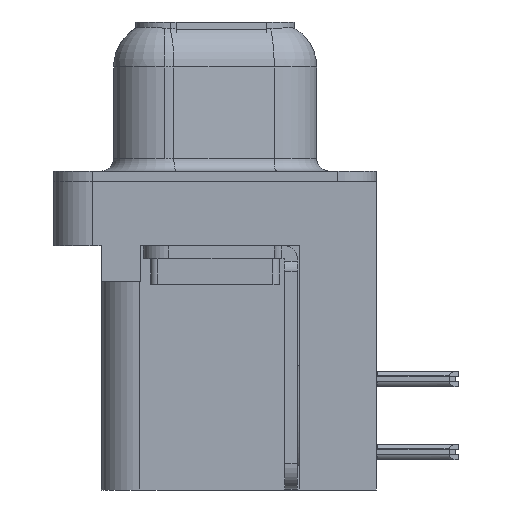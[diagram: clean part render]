
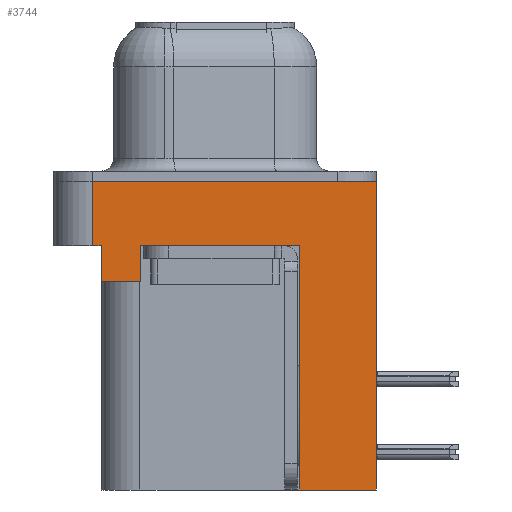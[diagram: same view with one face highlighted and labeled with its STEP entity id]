
A CAD part, left-side view. The second image highlights one B-rep face of the part: STEP entity #3744.
In plain terms, the highlighted planar face has unit normal (-1, 0, 0).
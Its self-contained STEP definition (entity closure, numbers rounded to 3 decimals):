
#469 = VERTEX_POINT ( 'NONE', #25335 ) ;
#672 = VERTEX_POINT ( 'NONE', #24510 ) ;
#760 = CARTESIAN_POINT ( 'NONE',  ( -3., -3.295, -12. ) ) ;
#1376 = CARTESIAN_POINT ( 'NONE',  ( -3., 4.775, -2.5 ) ) ;
#2022 = VECTOR ( 'NONE', #10264, 1000. ) ;
#2305 = LINE ( 'NONE', #1376, #24453 ) ;
#2306 = VECTOR ( 'NONE', #3288, 1000. ) ;
#2767 = LINE ( 'NONE', #17264, #2022 ) ;
#2804 = VERTEX_POINT ( 'NONE', #12885 ) ;
#3288 = DIRECTION ( 'NONE',  ( 0., 0., 1. ) ) ;
#3420 = EDGE_CURVE ( 'NONE', #29786, #469, #21900, .T. ) ;
#3744 = ADVANCED_FACE ( 'NONE', ( #12641 ), #6191, .T. ) ;
#4097 = ORIENTED_EDGE ( 'NONE', *, *, #20333, .F. ) ;
#4648 = CARTESIAN_POINT ( 'NONE',  ( -3., -3.295, -12. ) ) ;
#4680 = VERTEX_POINT ( 'NONE', #21486 ) ;
#5271 = LINE ( 'NONE', #19045, #11168 ) ;
#5850 = EDGE_CURVE ( 'NONE', #29208, #2804, #10130, .T. ) ;
#5971 = ORIENTED_EDGE ( 'NONE', *, *, #20144, .T. ) ;
#6191 = PLANE ( 'NONE',  #15124 ) ;
#6285 = ORIENTED_EDGE ( 'NONE', *, *, #27830, .T. ) ;
#8694 = DIRECTION ( 'NONE',  ( 0., 1., 0. ) ) ;
#8853 = ORIENTED_EDGE ( 'NONE', *, *, #11262, .F. ) ;
#8921 = VECTOR ( 'NONE', #8694, 1000. ) ;
#9347 = DIRECTION ( 'NONE',  ( 0., 0., 1. ) ) ;
#9670 = LINE ( 'NONE', #18084, #8921 ) ;
#10130 = LINE ( 'NONE', #19943, #10865 ) ;
#10264 = DIRECTION ( 'NONE',  ( 0., -1., 0. ) ) ;
#10350 = VERTEX_POINT ( 'NONE', #25648 ) ;
#10865 = VECTOR ( 'NONE', #22659, 1000. ) ;
#11033 = VERTEX_POINT ( 'NONE', #12132 ) ;
#11168 = VECTOR ( 'NONE', #9347, 1000. ) ;
#11219 = EDGE_CURVE ( 'NONE', #10350, #29208, #2305, .T. ) ;
#11262 = EDGE_CURVE ( 'NONE', #4680, #29013, #9670, .T. ) ;
#12012 = CARTESIAN_POINT ( 'NONE',  ( -3., -3.295, -2.5 ) ) ;
#12132 = CARTESIAN_POINT ( 'NONE',  ( -3., 4.425, -2.5 ) ) ;
#12162 = EDGE_LOOP ( 'NONE', ( #24472, #13879, #13935, #4097, #23419, #5971, #22652, #15176, #8853, #6285 ) ) ;
#12558 = CARTESIAN_POINT ( 'NONE',  ( -3., 2.895, -3.9 ) ) ;
#12641 = FACE_OUTER_BOUND ( 'NONE', #12162, .T. ) ;
#12758 = EDGE_CURVE ( 'NONE', #10350, #11033, #2767, .T. ) ;
#12885 = CARTESIAN_POINT ( 'NONE',  ( -3., -6.275, 0. ) ) ;
#13879 = ORIENTED_EDGE ( 'NONE', *, *, #11219, .F. ) ;
#13935 = ORIENTED_EDGE ( 'NONE', *, *, #12758, .T. ) ;
#14263 = DIRECTION ( 'NONE',  ( 0., 0., 1. ) ) ;
#15124 = AXIS2_PLACEMENT_3D ( 'NONE', #24739, #15525, #29367 ) ;
#15176 = ORIENTED_EDGE ( 'NONE', *, *, #24273, .F. ) ;
#15325 = DIRECTION ( 'NONE',  ( 0., 0., 1. ) ) ;
#15525 = DIRECTION ( 'NONE',  ( -1., 0., 0. ) ) ;
#15596 = LINE ( 'NONE', #4648, #21888 ) ;
#16414 = CARTESIAN_POINT ( 'NONE',  ( -3., 4.775, 0. ) ) ;
#17264 = CARTESIAN_POINT ( 'NONE',  ( -3., -6.275, -2.5 ) ) ;
#17925 = CARTESIAN_POINT ( 'NONE',  ( -3., -6.275, -2.5 ) ) ;
#18084 = CARTESIAN_POINT ( 'NONE',  ( -3., -3.295, -12. ) ) ;
#18569 = CARTESIAN_POINT ( 'NONE',  ( -3., 4.425, -3.9 ) ) ;
#19045 = CARTESIAN_POINT ( 'NONE',  ( -3., 2.895, -3.9 ) ) ;
#19943 = CARTESIAN_POINT ( 'NONE',  ( -3., -6.275, 0. ) ) ;
#20144 = EDGE_CURVE ( 'NONE', #29786, #672, #5271, .T. ) ;
#20255 = DIRECTION ( 'NONE',  ( 0., 0., 1. ) ) ;
#20333 = EDGE_CURVE ( 'NONE', #469, #11033, #24455, .T. ) ;
#20710 = VECTOR ( 'NONE', #27347, 1000. ) ;
#21486 = CARTESIAN_POINT ( 'NONE',  ( -3., -6.275, -12. ) ) ;
#21888 = VECTOR ( 'NONE', #14263, 1000. ) ;
#21900 = LINE ( 'NONE', #22704, #26707 ) ;
#22516 = DIRECTION ( 'NONE',  ( 0., 1., 0. ) ) ;
#22652 = ORIENTED_EDGE ( 'NONE', *, *, #25056, .T. ) ;
#22659 = DIRECTION ( 'NONE',  ( 0., -1., 0. ) ) ;
#22704 = CARTESIAN_POINT ( 'NONE',  ( -3., 4.425, -3.9 ) ) ;
#22854 = VECTOR ( 'NONE', #15325, 1000. ) ;
#23204 = LINE ( 'NONE', #17925, #22854 ) ;
#23419 = ORIENTED_EDGE ( 'NONE', *, *, #3420, .F. ) ;
#24273 = EDGE_CURVE ( 'NONE', #29013, #29406, #15596, .T. ) ;
#24453 = VECTOR ( 'NONE', #20255, 1000. ) ;
#24455 = LINE ( 'NONE', #18569, #2306 ) ;
#24472 = ORIENTED_EDGE ( 'NONE', *, *, #5850, .F. ) ;
#24510 = CARTESIAN_POINT ( 'NONE',  ( -3., 2.895, -2.5 ) ) ;
#24739 = CARTESIAN_POINT ( 'NONE',  ( -3., -6.275, -2.5 ) ) ;
#25056 = EDGE_CURVE ( 'NONE', #672, #29406, #26272, .T. ) ;
#25335 = CARTESIAN_POINT ( 'NONE',  ( -3., 4.425, -3.9 ) ) ;
#25648 = CARTESIAN_POINT ( 'NONE',  ( -3., 4.775, -2.5 ) ) ;
#26272 = LINE ( 'NONE', #27256, #20710 ) ;
#26707 = VECTOR ( 'NONE', #22516, 1000. ) ;
#27256 = CARTESIAN_POINT ( 'NONE',  ( -3., -6.275, -2.5 ) ) ;
#27347 = DIRECTION ( 'NONE',  ( 0., -1., 0. ) ) ;
#27830 = EDGE_CURVE ( 'NONE', #4680, #2804, #23204, .T. ) ;
#29013 = VERTEX_POINT ( 'NONE', #760 ) ;
#29208 = VERTEX_POINT ( 'NONE', #16414 ) ;
#29367 = DIRECTION ( 'NONE',  ( 0., 0., 1. ) ) ;
#29406 = VERTEX_POINT ( 'NONE', #12012 ) ;
#29786 = VERTEX_POINT ( 'NONE', #12558 ) ;
